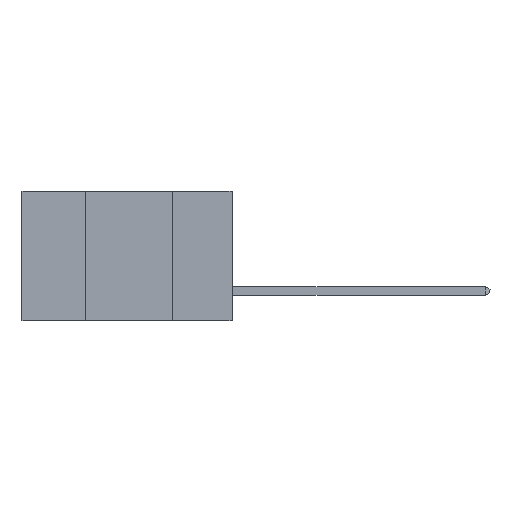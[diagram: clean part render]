
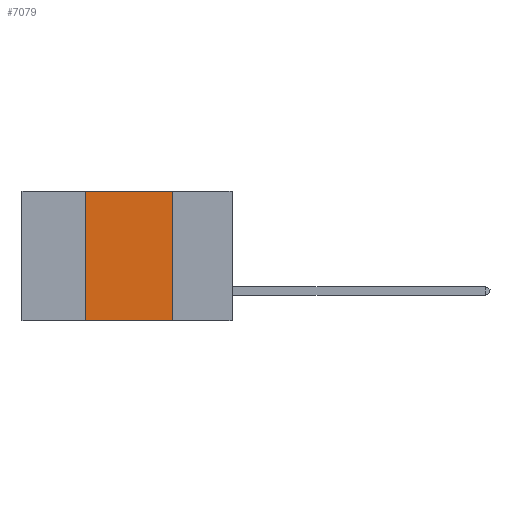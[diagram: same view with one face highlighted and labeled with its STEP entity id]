
A CAD part, left-side view. The second image highlights one B-rep face of the part: STEP entity #7079.
In plain terms, the highlighted planar face has unit normal (-1, 0, 0).
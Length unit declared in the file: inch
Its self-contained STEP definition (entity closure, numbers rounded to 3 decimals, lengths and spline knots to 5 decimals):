
#1178 = VECTOR ( 'NONE', #6644, 39.37008 ) ;
#1413 = DIRECTION ( 'NONE',  ( 1., 0., 0. ) ) ;
#1888 = AXIS2_PLACEMENT_3D ( 'NONE', #7093, #1413, #7993 ) ;
#2011 = EDGE_CURVE ( 'NONE', #4571, #9019, #4410, .T. ) ;
#2824 = VECTOR ( 'NONE', #10516, 39.37008 ) ;
#3072 = ORIENTED_EDGE ( 'NONE', *, *, #2011, .T. ) ;
#3242 = PLANE ( 'NONE',  #1888 ) ;
#3259 = CARTESIAN_POINT ( 'NONE',  ( 0., 0.6, -0.37 ) ) ;
#3811 = VECTOR ( 'NONE', #11673, 39.37008 ) ;
#3844 = DIRECTION ( 'NONE',  ( 0., 0., 1. ) ) ;
#3977 = CARTESIAN_POINT ( 'NONE',  ( 0., 0.17, -0.37 ) ) ;
#4207 = EDGE_CURVE ( 'NONE', #9709, #9019, #6702, .T. ) ;
#4410 = LINE ( 'NONE', #3259, #2824 ) ;
#4571 = VERTEX_POINT ( 'NONE', #7156 ) ;
#5177 = VECTOR ( 'NONE', #3844, 39.37008 ) ;
#5498 = CARTESIAN_POINT ( 'NONE',  ( 0., 0.17, 0. ) ) ;
#5975 = ORIENTED_EDGE ( 'NONE', *, *, #6570, .F. ) ;
#6274 = CARTESIAN_POINT ( 'NONE',  ( 0., 0.17, 0. ) ) ;
#6570 = EDGE_CURVE ( 'NONE', #7386, #9709, #10030, .T. ) ;
#6619 = CARTESIAN_POINT ( 'NONE',  ( 0., 0.42, 0. ) ) ;
#6644 = DIRECTION ( 'NONE',  ( 0., 0., -1. ) ) ;
#6702 = LINE ( 'NONE', #5498, #1178 ) ;
#7079 = ADVANCED_FACE ( 'NONE', ( #11473 ), #3242, .F. ) ;
#7093 = CARTESIAN_POINT ( 'NONE',  ( 0., 0.6, 0. ) ) ;
#7156 = CARTESIAN_POINT ( 'NONE',  ( 0., 0.42, -0.37 ) ) ;
#7386 = VERTEX_POINT ( 'NONE', #6619 ) ;
#7833 = CARTESIAN_POINT ( 'NONE',  ( 0., 0.6, 0. ) ) ;
#7993 = DIRECTION ( 'NONE',  ( 0., 0., -1. ) ) ;
#9019 = VERTEX_POINT ( 'NONE', #3977 ) ;
#9240 = EDGE_LOOP ( 'NONE', ( #9741, #5975, #10233, #3072 ) ) ;
#9329 = LINE ( 'NONE', #9563, #5177 ) ;
#9563 = CARTESIAN_POINT ( 'NONE',  ( 0., 0.42, 0. ) ) ;
#9709 = VERTEX_POINT ( 'NONE', #6274 ) ;
#9741 = ORIENTED_EDGE ( 'NONE', *, *, #4207, .F. ) ;
#10030 = LINE ( 'NONE', #7833, #3811 ) ;
#10233 = ORIENTED_EDGE ( 'NONE', *, *, #11339, .F. ) ;
#10516 = DIRECTION ( 'NONE',  ( 0., -1., 0. ) ) ;
#11339 = EDGE_CURVE ( 'NONE', #4571, #7386, #9329, .T. ) ;
#11473 = FACE_OUTER_BOUND ( 'NONE', #9240, .T. ) ;
#11673 = DIRECTION ( 'NONE',  ( 0., -1., 0. ) ) ;
